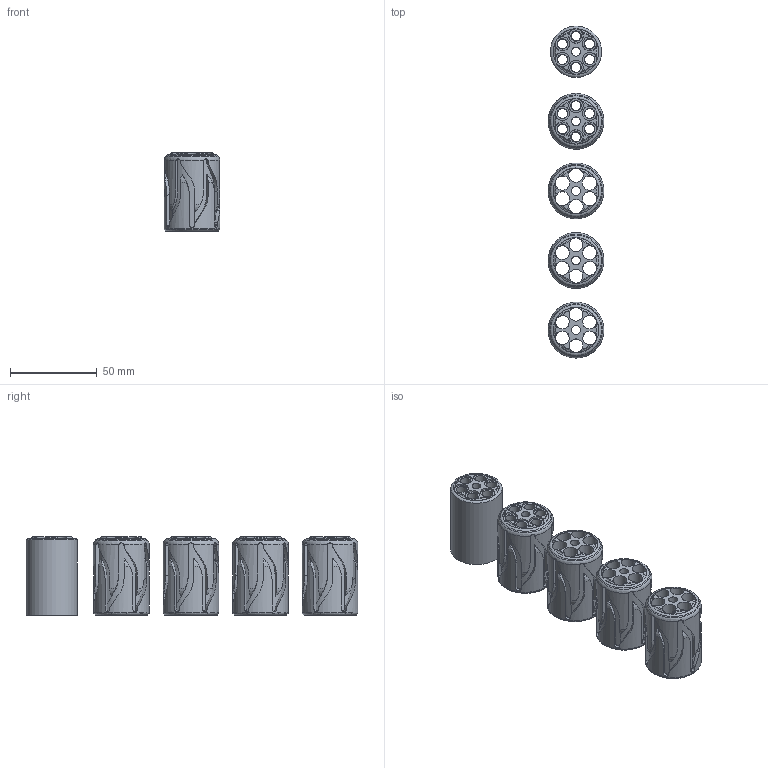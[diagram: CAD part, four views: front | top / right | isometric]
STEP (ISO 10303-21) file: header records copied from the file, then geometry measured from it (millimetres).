
FILE_DESCRIPTION(/* description */ (''),/* implementation_level */ '2;1');
FILE_NAME(/* name */ 'Cylinders.stp',/* time_stamp */ '2020-10-15T20:53:52-05:00',/* author */ (''),/* organization */ (''),/* preprocessor_version */ 'ST-DEVELOPER v15.2',/* originating_system */ 'Autodesk Translator Framework v2.0.0.5431',/* authorisation */ '');
FILE_SCHEMA (('AUTOMOTIVE_DESIGN { 1 0 10303 214 3 1 1 }'));
Length unit declared in the file: centimetre
Products named in the file (1): Cylinder
Bounding box: 32 x 190.75 x 45 mm (x, y, z)
Volume: 101165.5 mm3; surface area: 67036.6 mm2
Topology: 5 solids, 5 shells, 1355 faces, 3905 edges, 2547 vertices
Faces by surface type: bspline 524, cylinder 316, plane 267, cone 176, torus 72
Full cylindrical faces by diameter (mm): 5.1 x5, 6 x12, 7.8 x6, 8 x6, 8.2 x6, 29.5 x1, 32 x4
Entity records: 60069 total; most frequent: CARTESIAN_POINT 30646, ORIENTED_EDGE 7620, DIRECTION 3848, EDGE_CURVE 3810, VERTEX_POINT 2514, B_SPLINE_CURVE_WITH_KNOTS 2418, AXIS2_PLACEMENT_3D 1672, EDGE_LOOP 1474
